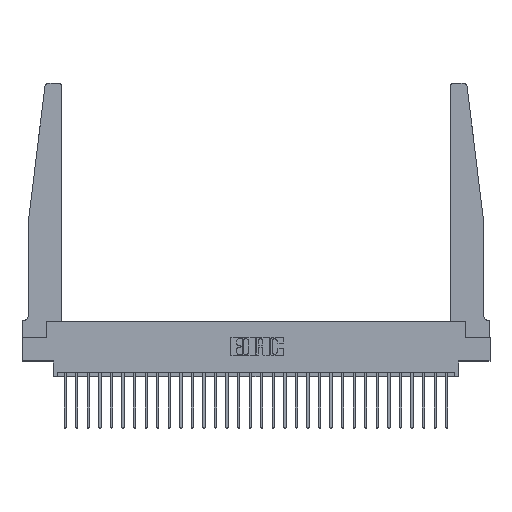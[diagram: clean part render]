
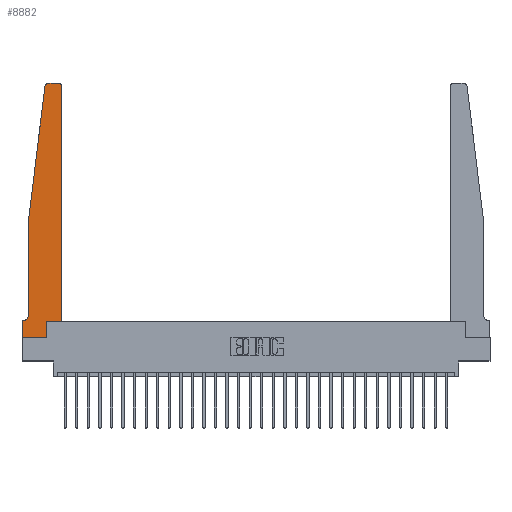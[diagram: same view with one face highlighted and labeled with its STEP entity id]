
A CAD part, top view. The second image highlights one B-rep face of the part: STEP entity #8882.
In plain terms, the highlighted planar face has unit normal (0, 0, 1).
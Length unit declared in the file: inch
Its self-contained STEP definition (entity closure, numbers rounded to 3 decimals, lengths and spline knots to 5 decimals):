
#72 = VECTOR ( 'NONE', #14206, 39.37008 ) ;
#249 = CARTESIAN_POINT ( 'NONE',  ( 0.065, 1.25, 0.37 ) ) ;
#900 = VERTEX_POINT ( 'NONE', #11726 ) ;
#979 = DIRECTION ( 'NONE',  ( -1., 0., 0. ) ) ;
#1378 = CARTESIAN_POINT ( 'NONE',  ( 0., 0., 0.37 ) ) ;
#1471 = LINE ( 'NONE', #27027, #27699 ) ;
#1488 = ORIENTED_EDGE ( 'NONE', *, *, #13688, .T. ) ;
#1763 = ORIENTED_EDGE ( 'NONE', *, *, #9238, .T. ) ;
#1970 = ORIENTED_EDGE ( 'NONE', *, *, #10314, .T. ) ;
#1988 = DIRECTION ( 'NONE',  ( 0., 0., 1. ) ) ;
#2146 = CARTESIAN_POINT ( 'NONE',  ( 0.2605, 0.18, 0.37 ) ) ;
#2385 = EDGE_CURVE ( 'NONE', #900, #3874, #11688, .T. ) ;
#2417 = AXIS2_PLACEMENT_3D ( 'NONE', #24953, #11900, #27121 ) ;
#2550 = VERTEX_POINT ( 'NONE', #14674 ) ;
#2894 = VERTEX_POINT ( 'NONE', #18097 ) ;
#3119 = ORIENTED_EDGE ( 'NONE', *, *, #2385, .T. ) ;
#3196 = EDGE_CURVE ( 'NONE', #22645, #900, #9245, .T. ) ;
#3198 = VERTEX_POINT ( 'NONE', #19144 ) ;
#3379 = AXIS2_PLACEMENT_3D ( 'NONE', #28091, #1988, #17235 ) ;
#3537 = VERTEX_POINT ( 'NONE', #7406 ) ;
#3578 = LINE ( 'NONE', #20031, #26098 ) ;
#3674 = EDGE_LOOP ( 'NONE', ( #22500, #19202, #1763, #1488, #19305, #27056, #27505, #18975, #1970, #21852, #3119, #15966 ) ) ;
#3874 = VERTEX_POINT ( 'NONE', #23673 ) ;
#5557 = EDGE_CURVE ( 'NONE', #26795, #2894, #14215, .T. ) ;
#6021 = EDGE_CURVE ( 'NONE', #2550, #26795, #9084, .T. ) ;
#6867 = CIRCLE ( 'NONE', #20936, 0.05 ) ;
#6874 = CARTESIAN_POINT ( 'NONE',  ( 0.015, 0.2375, 0.37 ) ) ;
#7406 = CARTESIAN_POINT ( 'NONE',  ( 0.2605, 0., 0.37 ) ) ;
#7638 = CARTESIAN_POINT ( 'NONE',  ( 0.425, 0.18, 0.37 ) ) ;
#8835 = CARTESIAN_POINT ( 'NONE',  ( 0., 0., 0.37 ) ) ;
#8882 = ADVANCED_FACE ( 'NONE', ( #20360 ), #12860, .T. ) ;
#9075 = DIRECTION ( 'NONE',  ( -1., 0., 0. ) ) ;
#9084 = LINE ( 'NONE', #11192, #26475 ) ;
#9238 = EDGE_CURVE ( 'NONE', #2894, #12668, #17978, .T. ) ;
#9245 = LINE ( 'NONE', #23521, #14350 ) ;
#9346 = CARTESIAN_POINT ( 'NONE',  ( 0.27653, 2.75, 0.37 ) ) ;
#9591 = DIRECTION ( 'NONE',  ( 1., 0., 0. ) ) ;
#9699 = EDGE_CURVE ( 'NONE', #20616, #19745, #25794, .T. ) ;
#10314 = EDGE_CURVE ( 'NONE', #3537, #22645, #3578, .T. ) ;
#10452 = DIRECTION ( 'NONE',  ( 1., 0., 0. ) ) ;
#10457 = DIRECTION ( 'NONE',  ( 1., 0., 0. ) ) ;
#11192 = CARTESIAN_POINT ( 'NONE',  ( 0.25, 2.75, 0.37 ) ) ;
#11286 = EDGE_CURVE ( 'NONE', #3874, #2550, #27395, .T. ) ;
#11545 = DIRECTION ( 'NONE',  ( -0.122, -0.992, 0. ) ) ;
#11688 = LINE ( 'NONE', #7638, #72 ) ;
#11726 = CARTESIAN_POINT ( 'NONE',  ( 0.425, 0.18, 0.37 ) ) ;
#11900 = DIRECTION ( 'NONE',  ( 0., 0., 1. ) ) ;
#12668 = VERTEX_POINT ( 'NONE', #249 ) ;
#12860 = PLANE ( 'NONE',  #3379 ) ;
#13019 = DIRECTION ( 'NONE',  ( 0., 0., 1. ) ) ;
#13498 = VECTOR ( 'NONE', #21888, 39.37008 ) ;
#13688 = EDGE_CURVE ( 'NONE', #12668, #18911, #14186, .T. ) ;
#14186 = LINE ( 'NONE', #18895, #25109 ) ;
#14206 = DIRECTION ( 'NONE',  ( 0., 1., 0. ) ) ;
#14215 = CIRCLE ( 'NONE', #2417, 0.03 ) ;
#14350 = VECTOR ( 'NONE', #10457, 39.37008 ) ;
#14674 = CARTESIAN_POINT ( 'NONE',  ( 0.395, 2.75, 0.37 ) ) ;
#15430 = EDGE_CURVE ( 'NONE', #19745, #3537, #1471, .T. ) ;
#15966 = ORIENTED_EDGE ( 'NONE', *, *, #11286, .T. ) ;
#17235 = DIRECTION ( 'NONE',  ( 1., 0., 0. ) ) ;
#17978 = LINE ( 'NONE', #24585, #23757 ) ;
#18097 = CARTESIAN_POINT ( 'NONE',  ( 0.24675, 2.72367, 0.37 ) ) ;
#18895 = CARTESIAN_POINT ( 'NONE',  ( 0.065, 1.25, 0.37 ) ) ;
#18911 = VERTEX_POINT ( 'NONE', #22297 ) ;
#18975 = ORIENTED_EDGE ( 'NONE', *, *, #15430, .T. ) ;
#19144 = CARTESIAN_POINT ( 'NONE',  ( 0.015, 0.1875, 0.37 ) ) ;
#19202 = ORIENTED_EDGE ( 'NONE', *, *, #5557, .T. ) ;
#19305 = ORIENTED_EDGE ( 'NONE', *, *, #23297, .T. ) ;
#19721 = CARTESIAN_POINT ( 'NONE',  ( 0., 0.1875, 0.37 ) ) ;
#19745 = VERTEX_POINT ( 'NONE', #1378 ) ;
#20031 = CARTESIAN_POINT ( 'NONE',  ( 0.2605, 0.18, 0.37 ) ) ;
#20360 = FACE_OUTER_BOUND ( 'NONE', #3674, .T. ) ;
#20616 = VERTEX_POINT ( 'NONE', #19721 ) ;
#20936 = AXIS2_PLACEMENT_3D ( 'NONE', #6874, #22132, #9075 ) ;
#21068 = DIRECTION ( 'NONE',  ( 0., -1., 0. ) ) ;
#21852 = ORIENTED_EDGE ( 'NONE', *, *, #3196, .T. ) ;
#21888 = DIRECTION ( 'NONE',  ( 0., -1., 0. ) ) ;
#22132 = DIRECTION ( 'NONE',  ( 0., 0., -1. ) ) ;
#22297 = CARTESIAN_POINT ( 'NONE',  ( 0.065, 0.2375, 0.37 ) ) ;
#22500 = ORIENTED_EDGE ( 'NONE', *, *, #6021, .T. ) ;
#22645 = VERTEX_POINT ( 'NONE', #2146 ) ;
#22725 = CARTESIAN_POINT ( 'NONE',  ( 0.065, 0.1875, 0.37 ) ) ;
#22735 = VECTOR ( 'NONE', #979, 39.37008 ) ;
#23297 = EDGE_CURVE ( 'NONE', #18911, #3198, #6867, .T. ) ;
#23411 = LINE ( 'NONE', #22725, #22735 ) ;
#23521 = CARTESIAN_POINT ( 'NONE',  ( 0.425, 0.18, 0.37 ) ) ;
#23673 = CARTESIAN_POINT ( 'NONE',  ( 0.425, 2.72, 0.37 ) ) ;
#23757 = VECTOR ( 'NONE', #11545, 39.37008 ) ;
#24585 = CARTESIAN_POINT ( 'NONE',  ( 0.065, 1.25, 0.37 ) ) ;
#24953 = CARTESIAN_POINT ( 'NONE',  ( 0.27653, 2.72, 0.37 ) ) ;
#24975 = AXIS2_PLACEMENT_3D ( 'NONE', #26092, #13019, #10452 ) ;
#25109 = VECTOR ( 'NONE', #21068, 39.37008 ) ;
#25794 = LINE ( 'NONE', #8835, #13498 ) ;
#26092 = CARTESIAN_POINT ( 'NONE',  ( 0.395, 2.72, 0.37 ) ) ;
#26098 = VECTOR ( 'NONE', #26520, 39.37008 ) ;
#26243 = EDGE_CURVE ( 'NONE', #3198, #20616, #23411, .T. ) ;
#26444 = DIRECTION ( 'NONE',  ( -1., 0., 0. ) ) ;
#26475 = VECTOR ( 'NONE', #26444, 39.37008 ) ;
#26520 = DIRECTION ( 'NONE',  ( 0., 1., 0. ) ) ;
#26795 = VERTEX_POINT ( 'NONE', #9346 ) ;
#27027 = CARTESIAN_POINT ( 'NONE',  ( 0., 0., 0.37 ) ) ;
#27056 = ORIENTED_EDGE ( 'NONE', *, *, #26243, .T. ) ;
#27121 = DIRECTION ( 'NONE',  ( 1., 0., 0. ) ) ;
#27395 = CIRCLE ( 'NONE', #24975, 0.03 ) ;
#27505 = ORIENTED_EDGE ( 'NONE', *, *, #9699, .T. ) ;
#27699 = VECTOR ( 'NONE', #9591, 39.37008 ) ;
#28091 = CARTESIAN_POINT ( 'NONE',  ( 0., 0.1875, 0.37 ) ) ;
